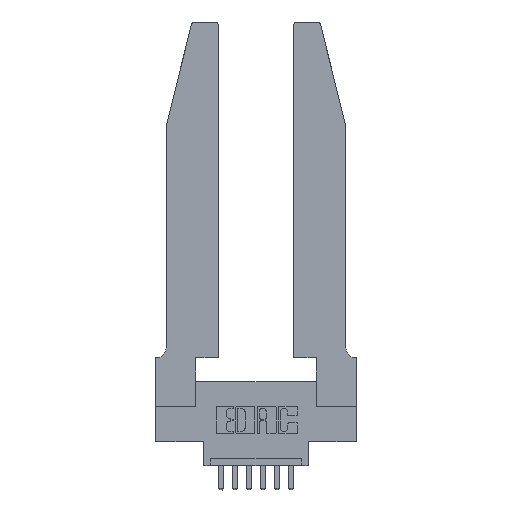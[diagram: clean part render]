
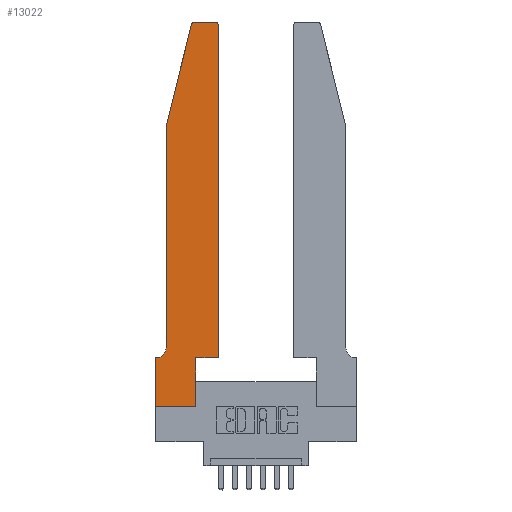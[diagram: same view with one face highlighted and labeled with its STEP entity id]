
A CAD part, top view. The second image highlights one B-rep face of the part: STEP entity #13022.
In plain terms, the highlighted planar face has unit normal (0, 0, 1).
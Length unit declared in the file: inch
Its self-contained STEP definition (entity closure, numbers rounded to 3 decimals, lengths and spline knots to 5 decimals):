
#3 = VECTOR ( 'NONE', #13613, 39.37008 ) ;
#103 = VECTOR ( 'NONE', #10219, 39.37008 ) ;
#649 = DIRECTION ( 'NONE',  ( -0.239, -0.971, 0. ) ) ;
#807 = DIRECTION ( 'NONE',  ( 1., 0., 0. ) ) ;
#840 = EDGE_CURVE ( 'NONE', #10787, #10900, #5999, .T. ) ;
#1083 = VECTOR ( 'NONE', #3336, 39.37008 ) ;
#1119 = DIRECTION ( 'NONE',  ( 1., 0., 0. ) ) ;
#1244 = LINE ( 'NONE', #12630, #6828 ) ;
#1267 = LINE ( 'NONE', #3507, #6691 ) ;
#1274 = LINE ( 'NONE', #3781, #5107 ) ;
#1320 = VERTEX_POINT ( 'NONE', #3730 ) ;
#1339 = EDGE_CURVE ( 'NONE', #14335, #13532, #1274, .T. ) ;
#1637 = LINE ( 'NONE', #3283, #1838 ) ;
#1838 = VECTOR ( 'NONE', #5531, 39.37008 ) ;
#1939 = CARTESIAN_POINT ( 'NONE',  ( 0.4205, 2.75, 0.37 ) ) ;
#2122 = CARTESIAN_POINT ( 'NONE',  ( 0.0755, 0.42, 0.37 ) ) ;
#2125 = LINE ( 'NONE', #3713, #3 ) ;
#2636 = EDGE_CURVE ( 'NONE', #10900, #7346, #9946, .T. ) ;
#2902 = EDGE_CURVE ( 'NONE', #4038, #7084, #1244, .T. ) ;
#2912 = DIRECTION ( 'NONE',  ( 0., 0., 1. ) ) ;
#3024 = DIRECTION ( 'NONE',  ( -1., 0., 0. ) ) ;
#3041 = CARTESIAN_POINT ( 'NONE',  ( 0.0755, 2., 0.37 ) ) ;
#3062 = AXIS2_PLACEMENT_3D ( 'NONE', #10992, #12079, #1119 ) ;
#3146 = AXIS2_PLACEMENT_3D ( 'NONE', #6811, #9110, #11294 ) ;
#3242 = EDGE_CURVE ( 'NONE', #7084, #1320, #4727, .T. ) ;
#3283 = CARTESIAN_POINT ( 'NONE',  ( 0.2865, 0.35, 0.37 ) ) ;
#3336 = DIRECTION ( 'NONE',  ( 0., -1., 0. ) ) ;
#3427 = CARTESIAN_POINT ( 'NONE',  ( 0., 0., 0.37 ) ) ;
#3444 = LINE ( 'NONE', #12479, #103 ) ;
#3507 = CARTESIAN_POINT ( 'NONE',  ( 0.0755, 2., 0.37 ) ) ;
#3713 = CARTESIAN_POINT ( 'NONE',  ( 0.2605, 2.75, 0.37 ) ) ;
#3730 = CARTESIAN_POINT ( 'NONE',  ( 0.4505, 2.72, 0.37 ) ) ;
#3781 = CARTESIAN_POINT ( 'NONE',  ( 0.0755, 2., 0.37 ) ) ;
#4038 = VERTEX_POINT ( 'NONE', #7301 ) ;
#4238 = ORIENTED_EDGE ( 'NONE', *, *, #8821, .T. ) ;
#4239 = PLANE ( 'NONE',  #12314 ) ;
#4727 = LINE ( 'NONE', #10973, #7520 ) ;
#4904 = CIRCLE ( 'NONE', #7243, 0.03 ) ;
#5107 = VECTOR ( 'NONE', #649, 39.37008 ) ;
#5204 = DIRECTION ( 'NONE',  ( 1., 0., 0. ) ) ;
#5531 = DIRECTION ( 'NONE',  ( 0., 1., 0. ) ) ;
#5748 = DIRECTION ( 'NONE',  ( 0., -1., 0. ) ) ;
#5785 = ORIENTED_EDGE ( 'NONE', *, *, #11202, .T. ) ;
#5999 = LINE ( 'NONE', #9700, #9622 ) ;
#6077 = ORIENTED_EDGE ( 'NONE', *, *, #3242, .T. ) ;
#6267 = VERTEX_POINT ( 'NONE', #9904 ) ;
#6418 = EDGE_CURVE ( 'NONE', #8730, #10787, #11228, .T. ) ;
#6486 = CARTESIAN_POINT ( 'NONE',  ( 0.0055, 0.35, 0.37 ) ) ;
#6675 = DIRECTION ( 'NONE',  ( 0., 1., 0. ) ) ;
#6691 = VECTOR ( 'NONE', #5748, 39.37008 ) ;
#6712 = VERTEX_POINT ( 'NONE', #9777 ) ;
#6802 = ORIENTED_EDGE ( 'NONE', *, *, #10336, .T. ) ;
#6811 = CARTESIAN_POINT ( 'NONE',  ( 0.0055, 0.42, 0.37 ) ) ;
#6828 = VECTOR ( 'NONE', #13692, 39.37008 ) ;
#6893 = EDGE_CURVE ( 'NONE', #6712, #4038, #1637, .T. ) ;
#7004 = CARTESIAN_POINT ( 'NONE',  ( 0.4505, 0.35, 0.37 ) ) ;
#7084 = VERTEX_POINT ( 'NONE', #7004 ) ;
#7098 = ORIENTED_EDGE ( 'NONE', *, *, #6418, .T. ) ;
#7243 = AXIS2_PLACEMENT_3D ( 'NONE', #12979, #2912, #5204 ) ;
#7301 = CARTESIAN_POINT ( 'NONE',  ( 0.2865, 0.35, 0.37 ) ) ;
#7346 = VERTEX_POINT ( 'NONE', #12467 ) ;
#7520 = VECTOR ( 'NONE', #6675, 39.37008 ) ;
#7532 = DIRECTION ( 'NONE',  ( 0., 0., 1. ) ) ;
#8245 = VERTEX_POINT ( 'NONE', #1939 ) ;
#8730 = VERTEX_POINT ( 'NONE', #2122 ) ;
#8814 = ORIENTED_EDGE ( 'NONE', *, *, #11652, .T. ) ;
#8821 = EDGE_CURVE ( 'NONE', #13532, #8730, #1267, .T. ) ;
#8990 = ORIENTED_EDGE ( 'NONE', *, *, #840, .T. ) ;
#9110 = DIRECTION ( 'NONE',  ( 0., 0., -1. ) ) ;
#9361 = ORIENTED_EDGE ( 'NONE', *, *, #6893, .T. ) ;
#9579 = CIRCLE ( 'NONE', #3062, 0.03 ) ;
#9622 = VECTOR ( 'NONE', #3024, 39.37008 ) ;
#9700 = CARTESIAN_POINT ( 'NONE',  ( 0.0755, 0.35, 0.37 ) ) ;
#9777 = CARTESIAN_POINT ( 'NONE',  ( 0.2865, 0., 0.37 ) ) ;
#9885 = CARTESIAN_POINT ( 'NONE',  ( 0., 0.35, 0.37 ) ) ;
#9904 = CARTESIAN_POINT ( 'NONE',  ( 0.284, 2.75, 0.37 ) ) ;
#9946 = LINE ( 'NONE', #3427, #1083 ) ;
#10080 = CARTESIAN_POINT ( 'NONE',  ( 0., 0.35, 0.37 ) ) ;
#10219 = DIRECTION ( 'NONE',  ( 1., 0., 0. ) ) ;
#10336 = EDGE_CURVE ( 'NONE', #1320, #8245, #9579, .T. ) ;
#10357 = ORIENTED_EDGE ( 'NONE', *, *, #13812, .T. ) ;
#10787 = VERTEX_POINT ( 'NONE', #6486 ) ;
#10900 = VERTEX_POINT ( 'NONE', #10080 ) ;
#10973 = CARTESIAN_POINT ( 'NONE',  ( 0.4505, 0.35, 0.37 ) ) ;
#10992 = CARTESIAN_POINT ( 'NONE',  ( 0.4205, 2.72, 0.37 ) ) ;
#11202 = EDGE_CURVE ( 'NONE', #6267, #14335, #4904, .T. ) ;
#11228 = CIRCLE ( 'NONE', #3146, 0.07 ) ;
#11294 = DIRECTION ( 'NONE',  ( -1., 0., 0. ) ) ;
#11652 = EDGE_CURVE ( 'NONE', #8245, #6267, #2125, .T. ) ;
#12079 = DIRECTION ( 'NONE',  ( 0., 0., 1. ) ) ;
#12121 = FACE_OUTER_BOUND ( 'NONE', #12494, .T. ) ;
#12314 = AXIS2_PLACEMENT_3D ( 'NONE', #9885, #7532, #807 ) ;
#12467 = CARTESIAN_POINT ( 'NONE',  ( 0., 0., 0.37 ) ) ;
#12479 = CARTESIAN_POINT ( 'NONE',  ( 0., 0., 0.37 ) ) ;
#12494 = EDGE_LOOP ( 'NONE', ( #8814, #5785, #12603, #4238, #7098, #8990, #13167, #10357, #9361, #13684, #6077, #6802 ) ) ;
#12603 = ORIENTED_EDGE ( 'NONE', *, *, #1339, .T. ) ;
#12630 = CARTESIAN_POINT ( 'NONE',  ( 0.4505, 0.35, 0.37 ) ) ;
#12979 = CARTESIAN_POINT ( 'NONE',  ( 0.284, 2.72, 0.37 ) ) ;
#13022 = ADVANCED_FACE ( 'NONE', ( #12121 ), #4239, .T. ) ;
#13167 = ORIENTED_EDGE ( 'NONE', *, *, #2636, .T. ) ;
#13476 = CARTESIAN_POINT ( 'NONE',  ( 0.25487, 2.72718, 0.37 ) ) ;
#13532 = VERTEX_POINT ( 'NONE', #3041 ) ;
#13613 = DIRECTION ( 'NONE',  ( -1., 0., 0. ) ) ;
#13684 = ORIENTED_EDGE ( 'NONE', *, *, #2902, .T. ) ;
#13692 = DIRECTION ( 'NONE',  ( 1., 0., 0. ) ) ;
#13812 = EDGE_CURVE ( 'NONE', #7346, #6712, #3444, .T. ) ;
#14335 = VERTEX_POINT ( 'NONE', #13476 ) ;
